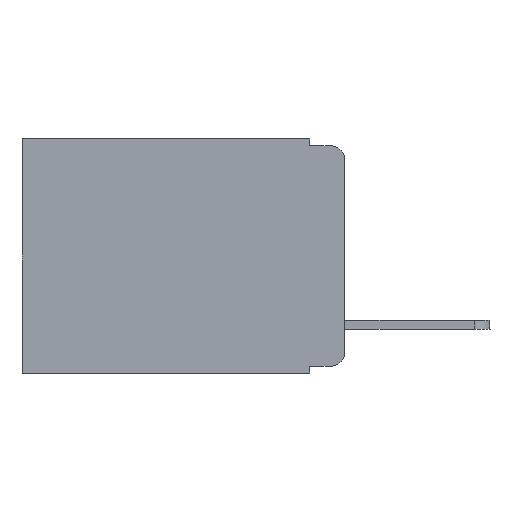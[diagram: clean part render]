
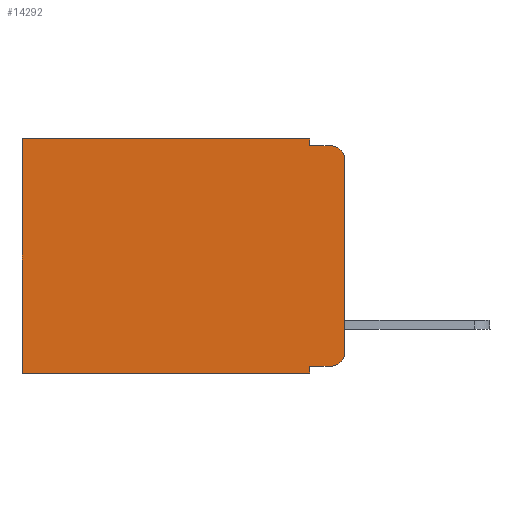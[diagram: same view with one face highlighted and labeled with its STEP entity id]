
A CAD part, left-side view. The second image highlights one B-rep face of the part: STEP entity #14292.
In plain terms, the highlighted planar face has unit normal (-1, 0, 0).
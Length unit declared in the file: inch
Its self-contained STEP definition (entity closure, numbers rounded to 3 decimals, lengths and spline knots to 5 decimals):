
#14 = LINE ( 'NONE', #4499, #6760 ) ;
#190 = LINE ( 'NONE', #6059, #213 ) ;
#213 = VECTOR ( 'NONE', #3582, 39.37008 ) ;
#444 = EDGE_CURVE ( 'NONE', #5075, #12800, #6375, .T. ) ;
#853 = VERTEX_POINT ( 'NONE', #2423 ) ;
#880 = VECTOR ( 'NONE', #3548, 39.37008 ) ;
#1169 = CARTESIAN_POINT ( 'NONE',  ( 0.298, 0.02, -0.01 ) ) ;
#1225 = CARTESIAN_POINT ( 'NONE',  ( 0.298, 0.473, -0.343 ) ) ;
#1536 = CARTESIAN_POINT ( 'NONE',  ( 0.298, 0.051, -0.333 ) ) ;
#1697 = ORIENTED_EDGE ( 'NONE', *, *, #13383, .F. ) ;
#1818 = DIRECTION ( 'NONE',  ( 0., 0., -1. ) ) ;
#1913 = VERTEX_POINT ( 'NONE', #1225 ) ;
#2324 = DIRECTION ( 'NONE',  ( 1., 0., 0. ) ) ;
#2423 = CARTESIAN_POINT ( 'NONE',  ( 0.298, 0.051, 0. ) ) ;
#2888 = VECTOR ( 'NONE', #4922, 39.37008 ) ;
#3108 = CARTESIAN_POINT ( 'NONE',  ( 0.298, 0., -0.343 ) ) ;
#3120 = EDGE_CURVE ( 'NONE', #4091, #11156, #5436, .T. ) ;
#3171 = VERTEX_POINT ( 'NONE', #8567 ) ;
#3206 = CARTESIAN_POINT ( 'NONE',  ( 0.298, 0., -0.03 ) ) ;
#3237 = VERTEX_POINT ( 'NONE', #6550 ) ;
#3290 = EDGE_CURVE ( 'NONE', #853, #3237, #9150, .T. ) ;
#3463 = DIRECTION ( 'NONE',  ( 0., 1., 0. ) ) ;
#3502 = AXIS2_PLACEMENT_3D ( 'NONE', #4094, #11837, #1818 ) ;
#3548 = DIRECTION ( 'NONE',  ( 0., 1., 0. ) ) ;
#3572 = ORIENTED_EDGE ( 'NONE', *, *, #14256, .T. ) ;
#3582 = DIRECTION ( 'NONE',  ( 0., 0., -1. ) ) ;
#3664 = EDGE_CURVE ( 'NONE', #3237, #1913, #190, .T. ) ;
#4091 = VERTEX_POINT ( 'NONE', #6794 ) ;
#4094 = CARTESIAN_POINT ( 'NONE',  ( 0.298, 0.02, -0.03 ) ) ;
#4199 = AXIS2_PLACEMENT_3D ( 'NONE', #5778, #2324, #6601 ) ;
#4338 = DIRECTION ( 'NONE',  ( 0., -1., 0. ) ) ;
#4477 = CARTESIAN_POINT ( 'NONE',  ( 0.298, 0.02, -0.333 ) ) ;
#4499 = CARTESIAN_POINT ( 'NONE',  ( 0.298, 0.051, 0. ) ) ;
#4681 = DIRECTION ( 'NONE',  ( -1., 0., 0. ) ) ;
#4809 = EDGE_CURVE ( 'NONE', #14345, #5075, #7130, .T. ) ;
#4922 = DIRECTION ( 'NONE',  ( 0., -1., 0. ) ) ;
#5075 = VERTEX_POINT ( 'NONE', #4477 ) ;
#5130 = PLANE ( 'NONE',  #4199 ) ;
#5207 = ORIENTED_EDGE ( 'NONE', *, *, #444, .T. ) ;
#5436 = LINE ( 'NONE', #13027, #12553 ) ;
#5515 = ORIENTED_EDGE ( 'NONE', *, *, #13719, .F. ) ;
#5688 = ORIENTED_EDGE ( 'NONE', *, *, #5940, .F. ) ;
#5728 = DIRECTION ( 'NONE',  ( 0., 0., -1. ) ) ;
#5778 = CARTESIAN_POINT ( 'NONE',  ( 0.298, 0., 0. ) ) ;
#5940 = EDGE_CURVE ( 'NONE', #9435, #12800, #9724, .T. ) ;
#6059 = CARTESIAN_POINT ( 'NONE',  ( 0.298, 0.473, 0. ) ) ;
#6274 = CARTESIAN_POINT ( 'NONE',  ( 0.298, 0.051, 0. ) ) ;
#6373 = ORIENTED_EDGE ( 'NONE', *, *, #12370, .F. ) ;
#6375 = CIRCLE ( 'NONE', #13345, 0.02 ) ;
#6467 = DIRECTION ( 'NONE',  ( 0., 0., -1. ) ) ;
#6550 = CARTESIAN_POINT ( 'NONE',  ( 0.298, 0.473, 0. ) ) ;
#6601 = DIRECTION ( 'NONE',  ( 0., 0., -1. ) ) ;
#6760 = VECTOR ( 'NONE', #5728, 39.37008 ) ;
#6794 = CARTESIAN_POINT ( 'NONE',  ( 0.298, 0.051, -0.01 ) ) ;
#7107 = CARTESIAN_POINT ( 'NONE',  ( 0.298, 0.02, -0.313 ) ) ;
#7130 = LINE ( 'NONE', #1536, #2888 ) ;
#7340 = ORIENTED_EDGE ( 'NONE', *, *, #4809, .T. ) ;
#7437 = DIRECTION ( 'NONE',  ( 0., 0., -1. ) ) ;
#7976 = CARTESIAN_POINT ( 'NONE',  ( 0.298, 0., -0.313 ) ) ;
#8513 = LINE ( 'NONE', #6274, #12552 ) ;
#8567 = CARTESIAN_POINT ( 'NONE',  ( 0.298, 0.051, -0.343 ) ) ;
#9074 = VECTOR ( 'NONE', #3463, 39.37008 ) ;
#9150 = LINE ( 'NONE', #10163, #880 ) ;
#9435 = VERTEX_POINT ( 'NONE', #3206 ) ;
#9724 = LINE ( 'NONE', #12070, #10053 ) ;
#9766 = CIRCLE ( 'NONE', #3502, 0.02 ) ;
#10053 = VECTOR ( 'NONE', #6467, 39.37008 ) ;
#10095 = LINE ( 'NONE', #3108, #9074 ) ;
#10163 = CARTESIAN_POINT ( 'NONE',  ( 0.298, 0., 0. ) ) ;
#10827 = ORIENTED_EDGE ( 'NONE', *, *, #3120, .F. ) ;
#10880 = FACE_OUTER_BOUND ( 'NONE', #14257, .T. ) ;
#11035 = CARTESIAN_POINT ( 'NONE',  ( 0.298, 0.051, -0.333 ) ) ;
#11156 = VERTEX_POINT ( 'NONE', #1169 ) ;
#11837 = DIRECTION ( 'NONE',  ( -1., 0., 0. ) ) ;
#12070 = CARTESIAN_POINT ( 'NONE',  ( 0.298, 0., 0. ) ) ;
#12370 = EDGE_CURVE ( 'NONE', #3171, #1913, #10095, .T. ) ;
#12552 = VECTOR ( 'NONE', #7437, 39.37008 ) ;
#12553 = VECTOR ( 'NONE', #4338, 39.37008 ) ;
#12800 = VERTEX_POINT ( 'NONE', #7976 ) ;
#13027 = CARTESIAN_POINT ( 'NONE',  ( 0.298, 0.051, -0.01 ) ) ;
#13345 = AXIS2_PLACEMENT_3D ( 'NONE', #7107, #4681, #13788 ) ;
#13383 = EDGE_CURVE ( 'NONE', #853, #4091, #14, .T. ) ;
#13399 = ORIENTED_EDGE ( 'NONE', *, *, #3290, .T. ) ;
#13719 = EDGE_CURVE ( 'NONE', #14345, #3171, #8513, .T. ) ;
#13788 = DIRECTION ( 'NONE',  ( 0., 0., -1. ) ) ;
#14061 = ORIENTED_EDGE ( 'NONE', *, *, #3664, .T. ) ;
#14256 = EDGE_CURVE ( 'NONE', #9435, #11156, #9766, .T. ) ;
#14257 = EDGE_LOOP ( 'NONE', ( #5688, #3572, #10827, #1697, #13399, #14061, #6373, #5515, #7340, #5207 ) ) ;
#14292 = ADVANCED_FACE ( 'NONE', ( #10880 ), #5130, .F. ) ;
#14345 = VERTEX_POINT ( 'NONE', #11035 ) ;
